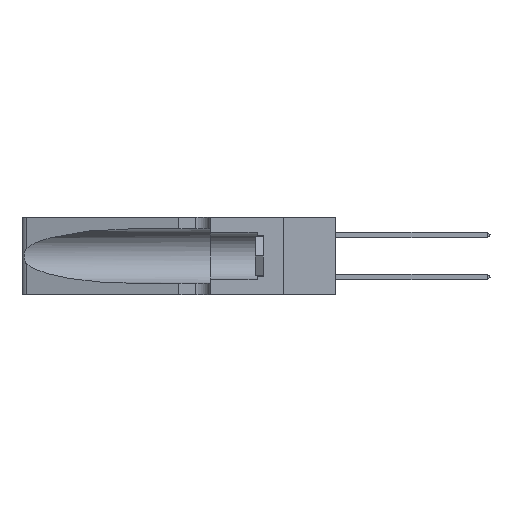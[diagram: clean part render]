
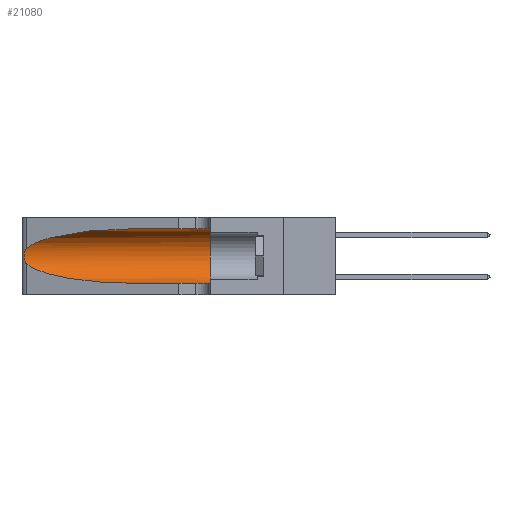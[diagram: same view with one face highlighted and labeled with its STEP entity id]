
A CAD part, left-side view. The second image highlights one B-rep face of the part: STEP entity #21080.
In plain terms, the highlighted cylindrical face has radius 3.308 mm (diameter 6.617 mm), a partial arc.
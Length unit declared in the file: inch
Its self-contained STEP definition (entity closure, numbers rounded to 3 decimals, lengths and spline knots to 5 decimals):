
#101 = ORIENTED_EDGE ( 'NONE', *, *, #39942, .T. ) ;
#423 = CARTESIAN_POINT ( 'NONE',  ( 0.25487, 1.22718, 0.22369 ) ) ;
#577 = CARTESIAN_POINT ( 'NONE',  ( 0.25639, 1.23186, 0.15144 ) ) ;
#1553 = VERTEX_POINT ( 'NONE', #3542 ) ;
#1558 = DIRECTION ( 'NONE',  ( 0., -1., 0. ) ) ;
#1895 = B_SPLINE_CURVE_WITH_KNOTS ( 'NONE', 3,
 ( #423, #36897, #7297, #30447, #10706, #33753, #14133, #37043, #17475, #40343, #20780, #577, #24072, #4040 ),
 .UNSPECIFIED., .F., .F.,
 ( 4, 2, 2, 2, 2, 2, 4 ),
 ( 0., 0.00027, 0.00053, 0.00107, 0.0016, 0.00187, 0.00214 ),
 .UNSPECIFIED. ) ;
#2611 = ORIENTED_EDGE ( 'NONE', *, *, #25314, .F. ) ;
#3081 = CARTESIAN_POINT ( 'NONE',  ( 0.1305, 1.61858, 0.05475 ) ) ;
#3542 = CARTESIAN_POINT ( 'NONE',  ( 0.1305, 0.35, 0.05475 ) ) ;
#4040 = CARTESIAN_POINT ( 'NONE',  ( 0.25487, 1.22718, 0.14631 ) ) ;
#4147 = CYLINDRICAL_SURFACE ( 'NONE', #42652, 0.13025 ) ;
#5074 = CARTESIAN_POINT ( 'NONE',  ( 0.1305, 0.72297, 0.31525 ) ) ;
#5231 = FACE_OUTER_BOUND ( 'NONE', #32489, .T. ) ;
#5267 = VERTEX_POINT ( 'NONE', #18810 ) ;
#5340 = VECTOR ( 'NONE', #23151, 39.37008 ) ;
#6349 = CARTESIAN_POINT ( 'NONE',  ( 0.1305, 0.72297, 0.31525 ) ) ;
#6997 = CARTESIAN_POINT ( 'NONE',  ( 0.1305, 0.35, 0.185 ) ) ;
#7297 = CARTESIAN_POINT ( 'NONE',  ( 0.25639, 1.23184, 0.21858 ) ) ;
#8053 = ORIENTED_EDGE ( 'NONE', *, *, #23888, .T. ) ;
#8730 = CARTESIAN_POINT ( 'NONE',  ( 0.25487, 1.22718, 0.14631 ) ) ;
#9723 = CARTESIAN_POINT ( 'NONE',  ( 0.18966, 0.96281, 0.31525 ) ) ;
#9840 = CIRCLE ( 'NONE', #32219, 0.13025 ) ;
#10408 = DIRECTION ( 'NONE',  ( 0., 0., 1. ) ) ;
#10706 = CARTESIAN_POINT ( 'NONE',  ( 0.25854, 1.2359, 0.20912 ) ) ;
#11238 = ORIENTED_EDGE ( 'NONE', *, *, #25568, .T. ) ;
#12160 = CARTESIAN_POINT ( 'NONE',  ( 0.2373, 1.15595, 0.08982 ) ) ;
#13155 = CARTESIAN_POINT ( 'NONE',  ( 0.25487, 1.22718, 0.22369 ) ) ;
#14133 = CARTESIAN_POINT ( 'NONE',  ( 0.26075, 1.23896, 0.19203 ) ) ;
#15092 = CARTESIAN_POINT ( 'NONE',  ( 0.1305, 1.61858, 0.31525 ) ) ;
#15547 = CARTESIAN_POINT ( 'NONE',  ( 0.1305, 0.72297, 0.05475 ) ) ;
#16766 = ORIENTED_EDGE ( 'NONE', *, *, #20580, .T. ) ;
#16970 = CARTESIAN_POINT ( 'NONE',  ( 0.1305, 0.72297, 0.05475 ) ) ;
#17475 = CARTESIAN_POINT ( 'NONE',  ( 0.26017, 1.23833, 0.17102 ) ) ;
#18785 = CARTESIAN_POINT ( 'NONE',  ( 0.1305, 1.61858, 0.185 ) ) ;
#18810 = CARTESIAN_POINT ( 'NONE',  ( 0.25487, 1.22718, 0.22369 ) ) ;
#19488 = ORIENTED_EDGE ( 'NONE', *, *, #41464, .F. ) ;
#20580 = EDGE_CURVE ( 'NONE', #5267, #34592, #1895, .T. ) ;
#20780 = CARTESIAN_POINT ( 'NONE',  ( 0.25789, 1.23486, 0.15765 ) ) ;
#21080 = ADVANCED_FACE ( 'NONE', ( #5231 ), #4147, .F. ) ;
#21951 = VERTEX_POINT ( 'NONE', #26159 ) ;
#22067 = DIRECTION ( 'NONE',  ( 0., 0., -1. ) ) ;
#22100 =( BOUNDED_CURVE ( )  B_SPLINE_CURVE ( 3, ( #6349, #9723, #32811, #13155 ),
 .UNSPECIFIED., .F., .T. ) 
 B_SPLINE_CURVE_WITH_KNOTS ( ( 4, 4 ),
 ( 1.5708, 2.84003 ),
 .UNSPECIFIED. ) 
 CURVE ( )  GEOMETRIC_REPRESENTATION_ITEM ( )  RATIONAL_B_SPLINE_CURVE ( ( 1., 0.87, 0.87, 1. ) ) 
 REPRESENTATION_ITEM ( '' )  );
#22110 = VERTEX_POINT ( 'NONE', #16970 ) ;
#23151 = DIRECTION ( 'NONE',  ( 0., -1., 0. ) ) ;
#23888 = EDGE_CURVE ( 'NONE', #22110, #1553, #30730, .T. ) ;
#24072 = CARTESIAN_POINT ( 'NONE',  ( 0.25555, 1.22993, 0.14849 ) ) ;
#24517 = LINE ( 'NONE', #15092, #25524 ) ;
#25314 = EDGE_CURVE ( 'NONE', #31776, #21951, #24517, .T. ) ;
#25524 = VECTOR ( 'NONE', #1558, 39.37008 ) ;
#25568 = EDGE_CURVE ( 'NONE', #31776, #5267, #22100, .T. ) ;
#26159 = CARTESIAN_POINT ( 'NONE',  ( 0.1305, 0.35, 0.31525 ) ) ;
#26557 =( BOUNDED_CURVE ( )  B_SPLINE_CURVE ( 3, ( #8730, #12160, #35153, #15547 ),
 .UNSPECIFIED., .F., .F. ) 
 B_SPLINE_CURVE_WITH_KNOTS ( ( 4, 4 ),
 ( 3.44316, 4.71239 ),
 .UNSPECIFIED. ) 
 CURVE ( )  GEOMETRIC_REPRESENTATION_ITEM ( )  RATIONAL_B_SPLINE_CURVE ( ( 1., 0.87, 0.87, 1. ) ) 
 REPRESENTATION_ITEM ( '' )  );
#30159 = DIRECTION ( 'NONE',  ( 0., 1., 0. ) ) ;
#30447 = CARTESIAN_POINT ( 'NONE',  ( 0.25787, 1.23484, 0.2124 ) ) ;
#30680 = CARTESIAN_POINT ( 'NONE',  ( 0.25487, 1.22718, 0.14631 ) ) ;
#30730 = LINE ( 'NONE', #3081, #5340 ) ;
#31776 = VERTEX_POINT ( 'NONE', #5074 ) ;
#32219 = AXIS2_PLACEMENT_3D ( 'NONE', #6997, #30159, #10408 ) ;
#32489 = EDGE_LOOP ( 'NONE', ( #11238, #16766, #101, #8053, #19488, #2611 ) ) ;
#32811 = CARTESIAN_POINT ( 'NONE',  ( 0.2373, 1.15595, 0.28018 ) ) ;
#33753 = CARTESIAN_POINT ( 'NONE',  ( 0.26018, 1.23835, 0.19895 ) ) ;
#34592 = VERTEX_POINT ( 'NONE', #30680 ) ;
#35153 = CARTESIAN_POINT ( 'NONE',  ( 0.18966, 0.96281, 0.05475 ) ) ;
#36897 = CARTESIAN_POINT ( 'NONE',  ( 0.25555, 1.22994, 0.2215 ) ) ;
#37043 = CARTESIAN_POINT ( 'NONE',  ( 0.26075, 1.23896, 0.178 ) ) ;
#38477 = DIRECTION ( 'NONE',  ( 0., -1., 0. ) ) ;
#39942 = EDGE_CURVE ( 'NONE', #34592, #22110, #26557, .T. ) ;
#40343 = CARTESIAN_POINT ( 'NONE',  ( 0.25856, 1.23593, 0.16098 ) ) ;
#41464 = EDGE_CURVE ( 'NONE', #21951, #1553, #9840, .T. ) ;
#42652 = AXIS2_PLACEMENT_3D ( 'NONE', #18785, #38477, #22067 ) ;
